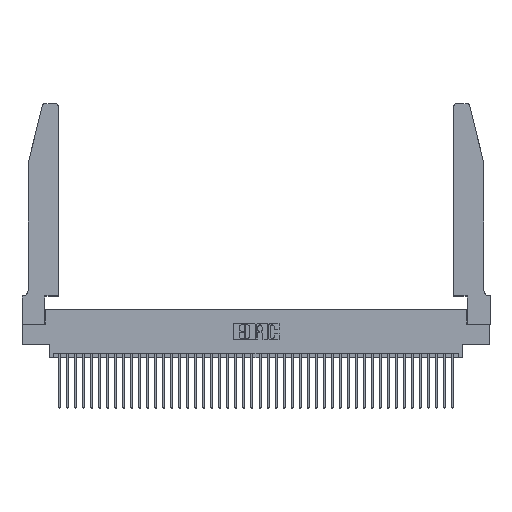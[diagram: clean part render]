
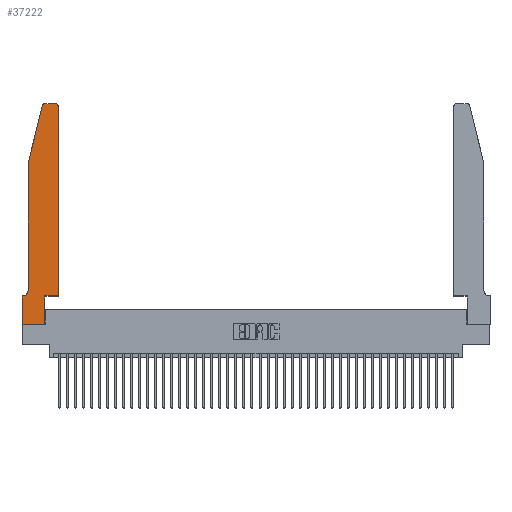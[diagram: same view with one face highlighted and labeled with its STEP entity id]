
A CAD part, top view. The second image highlights one B-rep face of the part: STEP entity #37222.
In plain terms, the highlighted planar face has unit normal (0, 0, 1).
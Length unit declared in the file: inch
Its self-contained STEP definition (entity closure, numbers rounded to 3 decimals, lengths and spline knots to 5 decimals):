
#771 = DIRECTION ( 'NONE',  ( 0., 0., 1. ) ) ;
#1485 = DIRECTION ( 'NONE',  ( -1., 0., 0. ) ) ;
#1497 = EDGE_CURVE ( 'NONE', #21379, #10370, #2136, .T. ) ;
#1519 = ORIENTED_EDGE ( 'NONE', *, *, #15440, .T. ) ;
#2136 = LINE ( 'NONE', #14788, #14134 ) ;
#2155 = CARTESIAN_POINT ( 'NONE',  ( 0., 0., 0.37 ) ) ;
#2937 = EDGE_CURVE ( 'NONE', #26232, #4536, #12972, .T. ) ;
#3202 = VERTEX_POINT ( 'NONE', #39255 ) ;
#4482 = VERTEX_POINT ( 'NONE', #13513 ) ;
#4500 = EDGE_CURVE ( 'NONE', #4536, #9554, #18543, .T. ) ;
#4536 = VERTEX_POINT ( 'NONE', #36252 ) ;
#5019 = VECTOR ( 'NONE', #35488, 39.37008 ) ;
#5072 = EDGE_CURVE ( 'NONE', #10370, #4482, #30979, .T. ) ;
#5090 = LINE ( 'NONE', #31083, #35317 ) ;
#5173 = AXIS2_PLACEMENT_3D ( 'NONE', #41291, #21481, #1485 ) ;
#5774 = CARTESIAN_POINT ( 'NONE',  ( 0.2865, 0.35, 0.37 ) ) ;
#6180 = VECTOR ( 'NONE', #38358, 39.37008 ) ;
#6463 = DIRECTION ( 'NONE',  ( 1., 0., 0. ) ) ;
#7735 = CARTESIAN_POINT ( 'NONE',  ( 0.0755, 0.42, 0.37 ) ) ;
#7758 = VERTEX_POINT ( 'NONE', #11263 ) ;
#8094 = ORIENTED_EDGE ( 'NONE', *, *, #27365, .T. ) ;
#8381 = FACE_OUTER_BOUND ( 'NONE', #16242, .T. ) ;
#8650 = EDGE_CURVE ( 'NONE', #4482, #26232, #41262, .T. ) ;
#8736 = CARTESIAN_POINT ( 'NONE',  ( 0.0755, 2., 0.37 ) ) ;
#9071 = DIRECTION ( 'NONE',  ( 0., 1., 0. ) ) ;
#9110 = VECTOR ( 'NONE', #38742, 39.37008 ) ;
#9554 = VERTEX_POINT ( 'NONE', #19515 ) ;
#10370 = VERTEX_POINT ( 'NONE', #34947 ) ;
#11109 = DIRECTION ( 'NONE',  ( -1., 0., 0. ) ) ;
#11263 = CARTESIAN_POINT ( 'NONE',  ( 0.0055, 0.35, 0.37 ) ) ;
#12014 = VERTEX_POINT ( 'NONE', #23015 ) ;
#12073 = CARTESIAN_POINT ( 'NONE',  ( 0.0755, 2., 0.37 ) ) ;
#12761 = CARTESIAN_POINT ( 'NONE',  ( 0.4205, 2.72, 0.37 ) ) ;
#12972 = LINE ( 'NONE', #14866, #6180 ) ;
#13513 = CARTESIAN_POINT ( 'NONE',  ( 0.4505, 2.72, 0.37 ) ) ;
#14134 = VECTOR ( 'NONE', #21488, 39.37008 ) ;
#14788 = CARTESIAN_POINT ( 'NONE',  ( 0.4505, 0.35, 0.37 ) ) ;
#14837 = DIRECTION ( 'NONE',  ( 0., -1., 0. ) ) ;
#14866 = CARTESIAN_POINT ( 'NONE',  ( 0.2605, 2.75, 0.37 ) ) ;
#15194 = CARTESIAN_POINT ( 'NONE',  ( 0.2865, 0.35, 0.37 ) ) ;
#15440 = EDGE_CURVE ( 'NONE', #35620, #7758, #24892, .T. ) ;
#15982 = EDGE_CURVE ( 'NONE', #20076, #21379, #20154, .T. ) ;
#16242 = EDGE_LOOP ( 'NONE', ( #25584, #39618, #17223, #30473, #1519, #8094, #34070, #26354, #29001, #28314, #32211, #24581 ) ) ;
#17033 = DIRECTION ( 'NONE',  ( 0., -1., 0. ) ) ;
#17223 = ORIENTED_EDGE ( 'NONE', *, *, #35779, .T. ) ;
#18543 = CIRCLE ( 'NONE', #40270, 0.03 ) ;
#19515 = CARTESIAN_POINT ( 'NONE',  ( 0.25487, 2.72718, 0.37 ) ) ;
#19594 = AXIS2_PLACEMENT_3D ( 'NONE', #12761, #42921, #6463 ) ;
#20076 = VERTEX_POINT ( 'NONE', #38711 ) ;
#20154 = LINE ( 'NONE', #5774, #5019 ) ;
#20526 = CARTESIAN_POINT ( 'NONE',  ( 0.0755, 2., 0.37 ) ) ;
#20546 = VECTOR ( 'NONE', #35268, 39.37008 ) ;
#21379 = VERTEX_POINT ( 'NONE', #15194 ) ;
#21481 = DIRECTION ( 'NONE',  ( 0., 0., -1. ) ) ;
#21488 = DIRECTION ( 'NONE',  ( 1., 0., 0. ) ) ;
#23015 = CARTESIAN_POINT ( 'NONE',  ( 0., 0., 0.37 ) ) ;
#24581 = ORIENTED_EDGE ( 'NONE', *, *, #8650, .T. ) ;
#24892 = CIRCLE ( 'NONE', #5173, 0.07 ) ;
#25321 = LINE ( 'NONE', #20526, #29533 ) ;
#25584 = ORIENTED_EDGE ( 'NONE', *, *, #2937, .T. ) ;
#26232 = VERTEX_POINT ( 'NONE', #36927 ) ;
#26354 = ORIENTED_EDGE ( 'NONE', *, *, #39918, .T. ) ;
#26469 = EDGE_CURVE ( 'NONE', #3202, #12014, #39496, .T. ) ;
#27135 = DIRECTION ( 'NONE',  ( 1., 0., 0. ) ) ;
#27262 = DIRECTION ( 'NONE',  ( 0., 0., 1. ) ) ;
#27365 = EDGE_CURVE ( 'NONE', #7758, #3202, #5090, .T. ) ;
#28290 = DIRECTION ( 'NONE',  ( 1., 0., 0. ) ) ;
#28314 = ORIENTED_EDGE ( 'NONE', *, *, #1497, .T. ) ;
#28410 = VECTOR ( 'NONE', #9071, 39.37008 ) ;
#28533 = EDGE_CURVE ( 'NONE', #35150, #35620, #25321, .T. ) ;
#29001 = ORIENTED_EDGE ( 'NONE', *, *, #15982, .T. ) ;
#29533 = VECTOR ( 'NONE', #17033, 39.37008 ) ;
#30473 = ORIENTED_EDGE ( 'NONE', *, *, #28533, .T. ) ;
#30641 = AXIS2_PLACEMENT_3D ( 'NONE', #33991, #27262, #27135 ) ;
#30979 = LINE ( 'NONE', #40928, #28410 ) ;
#31083 = CARTESIAN_POINT ( 'NONE',  ( 0.0755, 0.35, 0.37 ) ) ;
#31597 = CARTESIAN_POINT ( 'NONE',  ( 0., 0., 0.37 ) ) ;
#32211 = ORIENTED_EDGE ( 'NONE', *, *, #5072, .T. ) ;
#33991 = CARTESIAN_POINT ( 'NONE',  ( 0., 0.35, 0.37 ) ) ;
#34070 = ORIENTED_EDGE ( 'NONE', *, *, #26469, .T. ) ;
#34947 = CARTESIAN_POINT ( 'NONE',  ( 0.4505, 0.35, 0.37 ) ) ;
#35150 = VERTEX_POINT ( 'NONE', #12073 ) ;
#35268 = DIRECTION ( 'NONE',  ( -0.239, -0.971, 0. ) ) ;
#35317 = VECTOR ( 'NONE', #11109, 39.37008 ) ;
#35488 = DIRECTION ( 'NONE',  ( 0., 1., 0. ) ) ;
#35620 = VERTEX_POINT ( 'NONE', #7735 ) ;
#35702 = LINE ( 'NONE', #2155, #9110 ) ;
#35779 = EDGE_CURVE ( 'NONE', #9554, #35150, #38167, .T. ) ;
#36252 = CARTESIAN_POINT ( 'NONE',  ( 0.284, 2.75, 0.37 ) ) ;
#36927 = CARTESIAN_POINT ( 'NONE',  ( 0.4205, 2.75, 0.37 ) ) ;
#36983 = PLANE ( 'NONE',  #30641 ) ;
#37222 = ADVANCED_FACE ( 'NONE', ( #8381 ), #36983, .T. ) ;
#38167 = LINE ( 'NONE', #8736, #20546 ) ;
#38358 = DIRECTION ( 'NONE',  ( -1., 0., 0. ) ) ;
#38711 = CARTESIAN_POINT ( 'NONE',  ( 0.2865, 0., 0.37 ) ) ;
#38742 = DIRECTION ( 'NONE',  ( 1., 0., 0. ) ) ;
#39255 = CARTESIAN_POINT ( 'NONE',  ( 0., 0.35, 0.37 ) ) ;
#39496 = LINE ( 'NONE', #31597, #40013 ) ;
#39618 = ORIENTED_EDGE ( 'NONE', *, *, #4500, .T. ) ;
#39918 = EDGE_CURVE ( 'NONE', #12014, #20076, #35702, .T. ) ;
#40013 = VECTOR ( 'NONE', #14837, 39.37008 ) ;
#40270 = AXIS2_PLACEMENT_3D ( 'NONE', #41917, #771, #28290 ) ;
#40928 = CARTESIAN_POINT ( 'NONE',  ( 0.4505, 0.35, 0.37 ) ) ;
#41262 = CIRCLE ( 'NONE', #19594, 0.03 ) ;
#41291 = CARTESIAN_POINT ( 'NONE',  ( 0.0055, 0.42, 0.37 ) ) ;
#41917 = CARTESIAN_POINT ( 'NONE',  ( 0.284, 2.72, 0.37 ) ) ;
#42921 = DIRECTION ( 'NONE',  ( 0., 0., 1. ) ) ;
